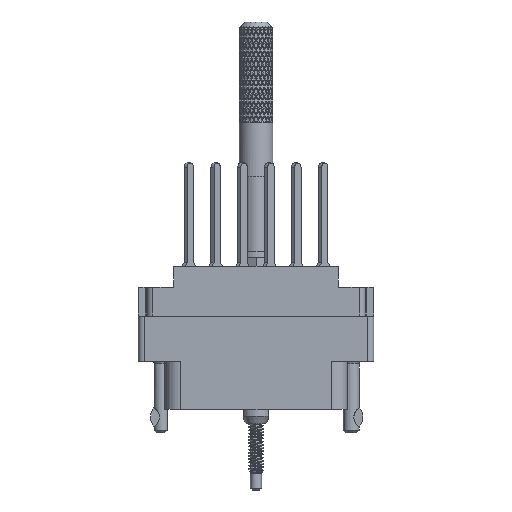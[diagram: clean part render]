
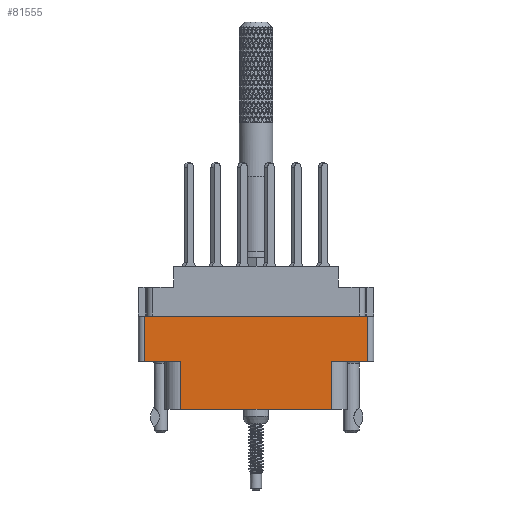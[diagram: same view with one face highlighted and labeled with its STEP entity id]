
A CAD part, front view. The second image highlights one B-rep face of the part: STEP entity #81555.
In plain terms, the highlighted planar face has unit normal (0, -1, 0).
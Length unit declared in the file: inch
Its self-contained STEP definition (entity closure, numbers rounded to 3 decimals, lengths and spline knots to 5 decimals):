
#3285 = VERTEX_POINT ( 'NONE', #106430 ) ;
#8806 = VECTOR ( 'NONE', #76362, 39.37008 ) ;
#9781 = CARTESIAN_POINT ( 'NONE',  ( -0.42, -0.343, -0.798 ) ) ;
#23395 = VECTOR ( 'NONE', #60383, 39.37008 ) ;
#23651 = EDGE_CURVE ( 'NONE', #127754, #146653, #55557, .T. ) ;
#25001 = LINE ( 'NONE', #106285, #8806 ) ;
#28305 = DIRECTION ( 'NONE',  ( 0., 0., -1. ) ) ;
#28429 = CARTESIAN_POINT ( 'NONE',  ( 0.624, -0.343, -0.277 ) ) ;
#29129 = ORIENTED_EDGE ( 'NONE', *, *, #78527, .T. ) ;
#31504 = CARTESIAN_POINT ( 'NONE',  ( 0., -0.343, -0.529 ) ) ;
#32266 = CARTESIAN_POINT ( 'NONE',  ( -0.42, -0.343, -0.529 ) ) ;
#32783 = ORIENTED_EDGE ( 'NONE', *, *, #140123, .F. ) ;
#34829 = CARTESIAN_POINT ( 'NONE',  ( 0.42, -0.343, -0.529 ) ) ;
#36729 = DIRECTION ( 'NONE',  ( 0., 0., 1. ) ) ;
#41858 = DIRECTION ( 'NONE',  ( 1., 0., 0. ) ) ;
#42673 = PLANE ( 'NONE',  #63411 ) ;
#47758 = DIRECTION ( 'NONE',  ( 1., 0., 0. ) ) ;
#51923 = EDGE_LOOP ( 'NONE', ( #29129, #69747, #163873, #32783, #120935, #145435, #73068, #147128 ) ) ;
#55557 = LINE ( 'NONE', #59429, #92849 ) ;
#57650 = VERTEX_POINT ( 'NONE', #151974 ) ;
#57852 = FACE_OUTER_BOUND ( 'NONE', #51923, .T. ) ;
#59429 = CARTESIAN_POINT ( 'NONE',  ( -0.656, -0.343, -0.277 ) ) ;
#60383 = DIRECTION ( 'NONE',  ( 0., 0., -1. ) ) ;
#60984 = LINE ( 'NONE', #63954, #177350 ) ;
#63411 = AXIS2_PLACEMENT_3D ( 'NONE', #132590, #74071, #146869 ) ;
#63954 = CARTESIAN_POINT ( 'NONE',  ( 0., -0.343, -0.529 ) ) ;
#65762 = VERTEX_POINT ( 'NONE', #9781 ) ;
#67894 = VERTEX_POINT ( 'NONE', #149132 ) ;
#69747 = ORIENTED_EDGE ( 'NONE', *, *, #184380, .T. ) ;
#73068 = ORIENTED_EDGE ( 'NONE', *, *, #149208, .F. ) ;
#74071 = DIRECTION ( 'NONE',  ( 0., -1., 0. ) ) ;
#76362 = DIRECTION ( 'NONE',  ( 0., 0., 1. ) ) ;
#78527 = EDGE_CURVE ( 'NONE', #136728, #65762, #142290, .T. ) ;
#79631 = EDGE_CURVE ( 'NONE', #92226, #3285, #141930, .T. ) ;
#81555 = ADVANCED_FACE ( 'NONE', ( #57852 ), #42673, .T. ) ;
#81699 = EDGE_CURVE ( 'NONE', #67894, #136728, #123078, .T. ) ;
#84226 = VECTOR ( 'NONE', #150333, 39.37008 ) ;
#85790 = VECTOR ( 'NONE', #47758, 39.37008 ) ;
#91196 = CARTESIAN_POINT ( 'NONE',  ( -0.42, -0.343, -0.529 ) ) ;
#92226 = VERTEX_POINT ( 'NONE', #183716 ) ;
#92849 = VECTOR ( 'NONE', #41858, 39.37008 ) ;
#98283 = CARTESIAN_POINT ( 'NONE',  ( -0.624, -0.343, -0.277 ) ) ;
#103439 = VECTOR ( 'NONE', #36729, 39.37008 ) ;
#105801 = LINE ( 'NONE', #109154, #103439 ) ;
#106285 = CARTESIAN_POINT ( 'NONE',  ( 0.624, -0.343, -0.798 ) ) ;
#106430 = CARTESIAN_POINT ( 'NONE',  ( 0.42, -0.343, -0.798 ) ) ;
#109154 = CARTESIAN_POINT ( 'NONE',  ( -0.624, -0.343, -0.798 ) ) ;
#120935 = ORIENTED_EDGE ( 'NONE', *, *, #157711, .T. ) ;
#123078 = LINE ( 'NONE', #31504, #85790 ) ;
#123770 = LINE ( 'NONE', #178382, #84226 ) ;
#127754 = VERTEX_POINT ( 'NONE', #98283 ) ;
#132590 = CARTESIAN_POINT ( 'NONE',  ( -0.624, -0.343, -0.798 ) ) ;
#136728 = VERTEX_POINT ( 'NONE', #91196 ) ;
#140123 = EDGE_CURVE ( 'NONE', #57650, #92226, #60984, .T. ) ;
#141930 = LINE ( 'NONE', #34829, #172178 ) ;
#142290 = LINE ( 'NONE', #32266, #23395 ) ;
#145435 = ORIENTED_EDGE ( 'NONE', *, *, #23651, .F. ) ;
#146653 = VERTEX_POINT ( 'NONE', #28429 ) ;
#146869 = DIRECTION ( 'NONE',  ( 0., 0., -1. ) ) ;
#147128 = ORIENTED_EDGE ( 'NONE', *, *, #81699, .T. ) ;
#149132 = CARTESIAN_POINT ( 'NONE',  ( -0.624, -0.343, -0.529 ) ) ;
#149208 = EDGE_CURVE ( 'NONE', #67894, #127754, #105801, .T. ) ;
#150333 = DIRECTION ( 'NONE',  ( 1., 0., 0. ) ) ;
#151974 = CARTESIAN_POINT ( 'NONE',  ( 0.624, -0.343, -0.529 ) ) ;
#157711 = EDGE_CURVE ( 'NONE', #57650, #146653, #25001, .T. ) ;
#163873 = ORIENTED_EDGE ( 'NONE', *, *, #79631, .F. ) ;
#166788 = DIRECTION ( 'NONE',  ( -1., 0., 0. ) ) ;
#172178 = VECTOR ( 'NONE', #28305, 39.37008 ) ;
#177350 = VECTOR ( 'NONE', #166788, 39.37008 ) ;
#178382 = CARTESIAN_POINT ( 'NONE',  ( -0.624, -0.343, -0.798 ) ) ;
#183716 = CARTESIAN_POINT ( 'NONE',  ( 0.42, -0.343, -0.529 ) ) ;
#184380 = EDGE_CURVE ( 'NONE', #65762, #3285, #123770, .T. ) ;
